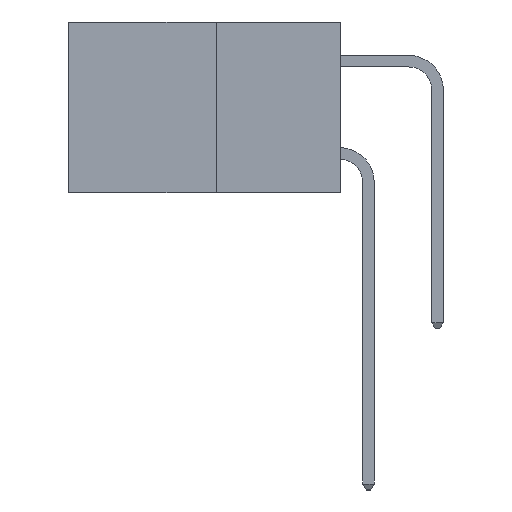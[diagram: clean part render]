
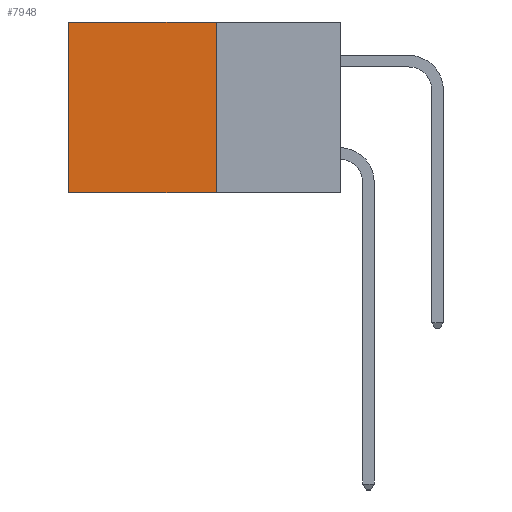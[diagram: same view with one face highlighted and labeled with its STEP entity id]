
A CAD part, left-side view. The second image highlights one B-rep face of the part: STEP entity #7948.
In plain terms, the highlighted planar face has unit normal (-1, 0, 0).
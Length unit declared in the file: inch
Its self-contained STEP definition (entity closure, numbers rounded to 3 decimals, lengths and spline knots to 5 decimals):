
#1660 = VERTEX_POINT ( 'NONE', #10517 ) ;
#1676 = AXIS2_PLACEMENT_3D ( 'NONE', #3655, #3766, #3728 ) ;
#1791 = CARTESIAN_POINT ( 'NONE',  ( 0.277, 0.27, 0. ) ) ;
#1854 = VECTOR ( 'NONE', #9077, 39.37008 ) ;
#2042 = VECTOR ( 'NONE', #9977, 39.37008 ) ;
#2124 = DIRECTION ( 'NONE',  ( 0., 1., 0. ) ) ;
#2199 = CARTESIAN_POINT ( 'NONE',  ( 0.277, 0.27, -0.37 ) ) ;
#2425 = PLANE ( 'NONE',  #1676 ) ;
#2696 = EDGE_CURVE ( 'NONE', #6348, #4071, #10561, .T. ) ;
#3655 = CARTESIAN_POINT ( 'NONE',  ( 0.277, 0.27, -0.37 ) ) ;
#3728 = DIRECTION ( 'NONE',  ( 0., 0., -1. ) ) ;
#3766 = DIRECTION ( 'NONE',  ( 1., 0., 0. ) ) ;
#4071 = VERTEX_POINT ( 'NONE', #8468 ) ;
#4158 = LINE ( 'NONE', #8195, #1854 ) ;
#4448 = VECTOR ( 'NONE', #6708, 39.37008 ) ;
#4836 = ORIENTED_EDGE ( 'NONE', *, *, #8862, .F. ) ;
#4848 = ORIENTED_EDGE ( 'NONE', *, *, #5404, .T. ) ;
#4885 = CARTESIAN_POINT ( 'NONE',  ( 0.277, 0.27, 0. ) ) ;
#5024 = LINE ( 'NONE', #2199, #7565 ) ;
#5404 = EDGE_CURVE ( 'NONE', #6348, #7634, #6987, .T. ) ;
#6348 = VERTEX_POINT ( 'NONE', #1791 ) ;
#6404 = EDGE_LOOP ( 'NONE', ( #9137, #4836, #9682, #4848 ) ) ;
#6708 = DIRECTION ( 'NONE',  ( 0., 1., 0. ) ) ;
#6900 = CARTESIAN_POINT ( 'NONE',  ( 0.277, 0.27, -0.37 ) ) ;
#6987 = LINE ( 'NONE', #4885, #4448 ) ;
#7438 = CARTESIAN_POINT ( 'NONE',  ( 0.277, 0.59, 0. ) ) ;
#7565 = VECTOR ( 'NONE', #2124, 39.37008 ) ;
#7634 = VERTEX_POINT ( 'NONE', #7438 ) ;
#7948 = ADVANCED_FACE ( 'NONE', ( #9356 ), #2425, .F. ) ;
#8195 = CARTESIAN_POINT ( 'NONE',  ( 0.277, 0.59, -0.37 ) ) ;
#8468 = CARTESIAN_POINT ( 'NONE',  ( 0.277, 0.27, -0.37 ) ) ;
#8862 = EDGE_CURVE ( 'NONE', #4071, #1660, #5024, .T. ) ;
#9077 = DIRECTION ( 'NONE',  ( 0., 0., -1. ) ) ;
#9137 = ORIENTED_EDGE ( 'NONE', *, *, #10048, .T. ) ;
#9356 = FACE_OUTER_BOUND ( 'NONE', #6404, .T. ) ;
#9682 = ORIENTED_EDGE ( 'NONE', *, *, #2696, .F. ) ;
#9977 = DIRECTION ( 'NONE',  ( 0., 0., -1. ) ) ;
#10048 = EDGE_CURVE ( 'NONE', #7634, #1660, #4158, .T. ) ;
#10517 = CARTESIAN_POINT ( 'NONE',  ( 0.277, 0.59, -0.37 ) ) ;
#10561 = LINE ( 'NONE', #6900, #2042 ) ;
